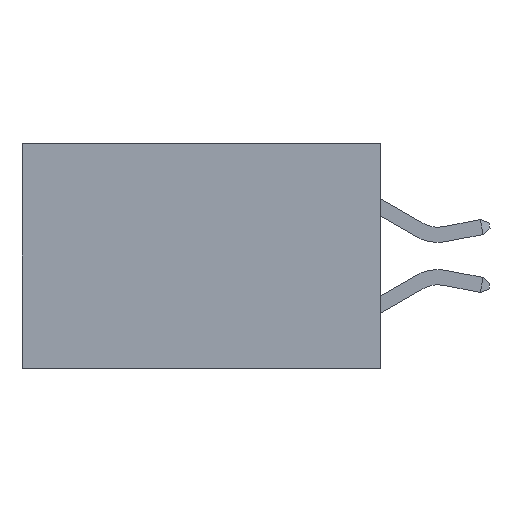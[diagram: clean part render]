
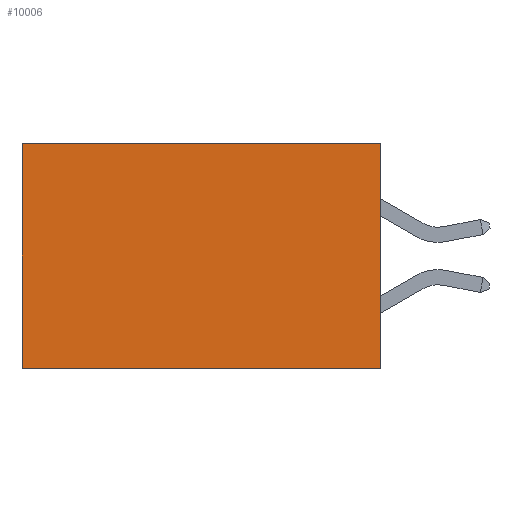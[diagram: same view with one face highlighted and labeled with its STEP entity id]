
A CAD part, left-side view. The second image highlights one B-rep face of the part: STEP entity #10006.
In plain terms, the highlighted planar face has unit normal (-1, 0, 0).
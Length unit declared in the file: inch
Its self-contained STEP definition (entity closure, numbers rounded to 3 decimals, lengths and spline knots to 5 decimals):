
#321 = ORIENTED_EDGE ( 'NONE', *, *, #3011, .F. ) ;
#1359 = LINE ( 'NONE', #14714, #7860 ) ;
#1458 = VECTOR ( 'NONE', #2160, 39.37008 ) ;
#1604 = EDGE_CURVE ( 'NONE', #14718, #4736, #8756, .T. ) ;
#2160 = DIRECTION ( 'NONE',  ( 0., 0., -1. ) ) ;
#2341 = VERTEX_POINT ( 'NONE', #16244 ) ;
#3011 = EDGE_CURVE ( 'NONE', #9596, #2341, #10920, .T. ) ;
#3886 = DIRECTION ( 'NONE',  ( 0., 0., -1. ) ) ;
#4113 = DIRECTION ( 'NONE',  ( 1., 0., 0. ) ) ;
#4211 = CARTESIAN_POINT ( 'NONE',  ( 0.277, 0.59, 0. ) ) ;
#4736 = VERTEX_POINT ( 'NONE', #15759 ) ;
#5455 = EDGE_CURVE ( 'NONE', #9596, #14718, #12029, .T. ) ;
#7304 = CARTESIAN_POINT ( 'NONE',  ( 0.277, 0., 0. ) ) ;
#7504 = VECTOR ( 'NONE', #3886, 39.37008 ) ;
#7860 = VECTOR ( 'NONE', #13448, 39.37008 ) ;
#8170 = CARTESIAN_POINT ( 'NONE',  ( 0.277, 0.59, -0.37 ) ) ;
#8659 = VECTOR ( 'NONE', #8767, 39.37008 ) ;
#8756 = LINE ( 'NONE', #8170, #1458 ) ;
#8767 = DIRECTION ( 'NONE',  ( 0., 1., 0. ) ) ;
#9596 = VERTEX_POINT ( 'NONE', #7304 ) ;
#10006 = ADVANCED_FACE ( 'NONE', ( #11790 ), #11808, .F. ) ;
#10549 = CARTESIAN_POINT ( 'NONE',  ( 0.277, 0., 0. ) ) ;
#10555 = CARTESIAN_POINT ( 'NONE',  ( 0.277, 0., -0.37 ) ) ;
#10920 = LINE ( 'NONE', #12302, #7504 ) ;
#11790 = FACE_OUTER_BOUND ( 'NONE', #12207, .T. ) ;
#11808 = PLANE ( 'NONE',  #15005 ) ;
#12029 = LINE ( 'NONE', #10549, #8659 ) ;
#12207 = EDGE_LOOP ( 'NONE', ( #14993, #14320, #321, #14525 ) ) ;
#12302 = CARTESIAN_POINT ( 'NONE',  ( 0.277, 0., -0.37 ) ) ;
#13081 = DIRECTION ( 'NONE',  ( 0., 0., -1. ) ) ;
#13448 = DIRECTION ( 'NONE',  ( 0., 1., 0. ) ) ;
#14320 = ORIENTED_EDGE ( 'NONE', *, *, #15105, .F. ) ;
#14525 = ORIENTED_EDGE ( 'NONE', *, *, #5455, .T. ) ;
#14714 = CARTESIAN_POINT ( 'NONE',  ( 0.277, 0., -0.37 ) ) ;
#14718 = VERTEX_POINT ( 'NONE', #4211 ) ;
#14993 = ORIENTED_EDGE ( 'NONE', *, *, #1604, .T. ) ;
#15005 = AXIS2_PLACEMENT_3D ( 'NONE', #10555, #4113, #13081 ) ;
#15105 = EDGE_CURVE ( 'NONE', #2341, #4736, #1359, .T. ) ;
#15759 = CARTESIAN_POINT ( 'NONE',  ( 0.277, 0.59, -0.37 ) ) ;
#16244 = CARTESIAN_POINT ( 'NONE',  ( 0.277, 0., -0.37 ) ) ;
